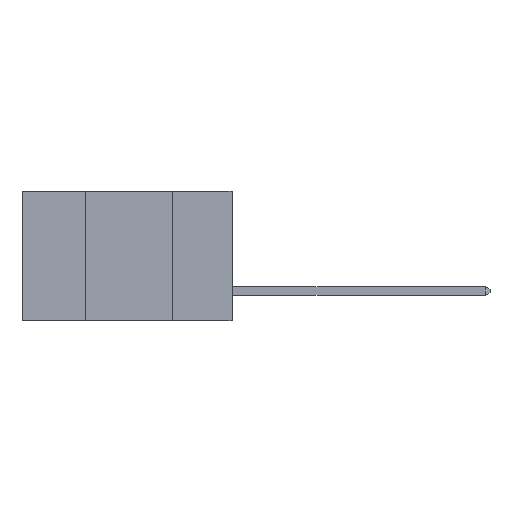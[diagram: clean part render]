
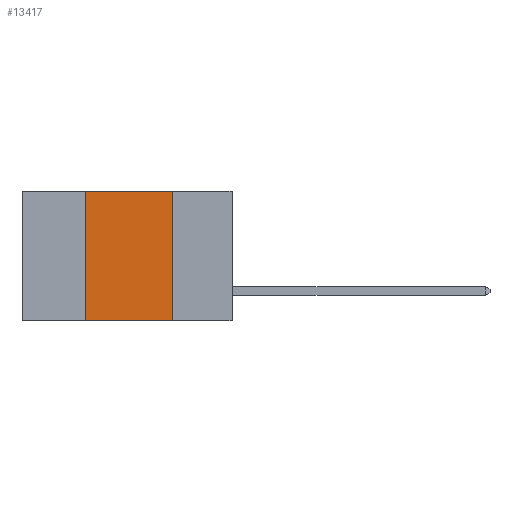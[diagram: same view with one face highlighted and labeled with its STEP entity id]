
A CAD part, left-side view. The second image highlights one B-rep face of the part: STEP entity #13417.
In plain terms, the highlighted planar face has unit normal (-1, 0, 0).
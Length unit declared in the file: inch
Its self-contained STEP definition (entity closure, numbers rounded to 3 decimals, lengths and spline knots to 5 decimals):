
#24 = VERTEX_POINT ( 'NONE', #11763 ) ;
#111 = VERTEX_POINT ( 'NONE', #4248 ) ;
#918 = CARTESIAN_POINT ( 'NONE',  ( 0., 0.17, 0. ) ) ;
#974 = ORIENTED_EDGE ( 'NONE', *, *, #14668, .T. ) ;
#1540 = EDGE_CURVE ( 'NONE', #6791, #13652, #6371, .T. ) ;
#2558 = CARTESIAN_POINT ( 'NONE',  ( 0., 0.6, 0. ) ) ;
#2753 = FACE_OUTER_BOUND ( 'NONE', #10821, .T. ) ;
#2831 = VECTOR ( 'NONE', #13075, 39.37008 ) ;
#2926 = CARTESIAN_POINT ( 'NONE',  ( 0., 0.17, 0. ) ) ;
#3083 = AXIS2_PLACEMENT_3D ( 'NONE', #16813, #4072, #13150 ) ;
#3458 = CARTESIAN_POINT ( 'NONE',  ( 0., 0.6, -0.37 ) ) ;
#3964 = VECTOR ( 'NONE', #7827, 39.37008 ) ;
#4072 = DIRECTION ( 'NONE',  ( 1., 0., 0. ) ) ;
#4248 = CARTESIAN_POINT ( 'NONE',  ( 0., 0.42, 0. ) ) ;
#6371 = LINE ( 'NONE', #2926, #2831 ) ;
#6791 = VERTEX_POINT ( 'NONE', #918 ) ;
#7099 = ORIENTED_EDGE ( 'NONE', *, *, #15520, .F. ) ;
#7243 = CARTESIAN_POINT ( 'NONE',  ( 0., 0.17, -0.37 ) ) ;
#7827 = DIRECTION ( 'NONE',  ( 0., -1., 0. ) ) ;
#7905 = VECTOR ( 'NONE', #14245, 39.37008 ) ;
#8224 = ORIENTED_EDGE ( 'NONE', *, *, #1540, .F. ) ;
#8653 = EDGE_CURVE ( 'NONE', #111, #6791, #10876, .T. ) ;
#10545 = PLANE ( 'NONE',  #3083 ) ;
#10821 = EDGE_LOOP ( 'NONE', ( #8224, #11248, #7099, #974 ) ) ;
#10876 = LINE ( 'NONE', #2558, #3964 ) ;
#11248 = ORIENTED_EDGE ( 'NONE', *, *, #8653, .F. ) ;
#11763 = CARTESIAN_POINT ( 'NONE',  ( 0., 0.42, -0.37 ) ) ;
#12976 = CARTESIAN_POINT ( 'NONE',  ( 0., 0.42, 0. ) ) ;
#13075 = DIRECTION ( 'NONE',  ( 0., 0., -1. ) ) ;
#13150 = DIRECTION ( 'NONE',  ( 0., 0., -1. ) ) ;
#13417 = ADVANCED_FACE ( 'NONE', ( #2753 ), #10545, .F. ) ;
#13652 = VERTEX_POINT ( 'NONE', #7243 ) ;
#13832 = DIRECTION ( 'NONE',  ( 0., -1., 0. ) ) ;
#14245 = DIRECTION ( 'NONE',  ( 0., 0., 1. ) ) ;
#14668 = EDGE_CURVE ( 'NONE', #24, #13652, #15885, .T. ) ;
#14683 = LINE ( 'NONE', #12976, #7905 ) ;
#15513 = VECTOR ( 'NONE', #13832, 39.37008 ) ;
#15520 = EDGE_CURVE ( 'NONE', #24, #111, #14683, .T. ) ;
#15885 = LINE ( 'NONE', #3458, #15513 ) ;
#16813 = CARTESIAN_POINT ( 'NONE',  ( 0., 0.6, 0. ) ) ;
